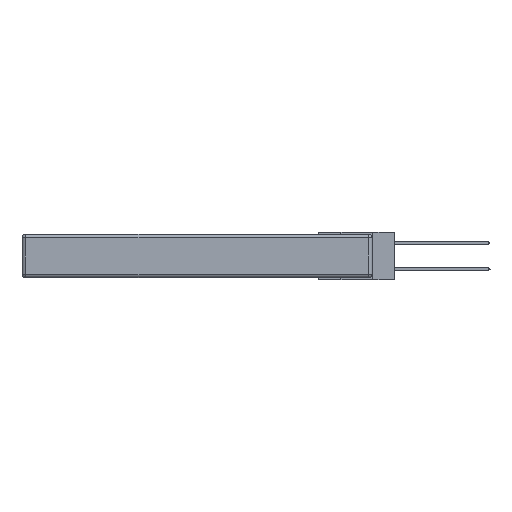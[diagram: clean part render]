
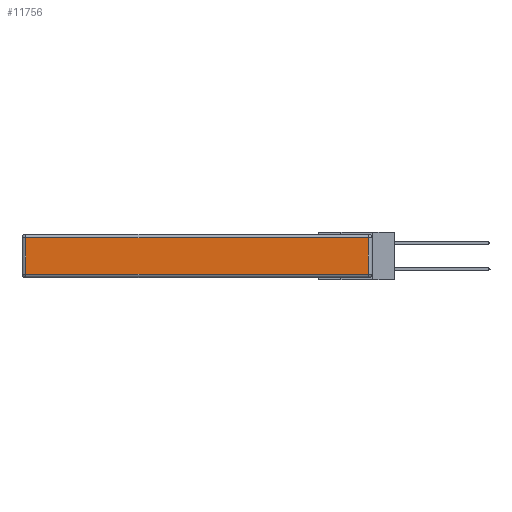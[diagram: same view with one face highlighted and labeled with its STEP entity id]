
A CAD part, left-side view. The second image highlights one B-rep face of the part: STEP entity #11756.
In plain terms, the highlighted planar face has unit normal (-1, 0, 0).
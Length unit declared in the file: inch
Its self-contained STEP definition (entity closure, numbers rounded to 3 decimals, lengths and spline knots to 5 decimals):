
#419 = ORIENTED_EDGE ( 'NONE', *, *, #9280, .T. ) ;
#491 = CARTESIAN_POINT ( 'NONE',  ( 0., 0.03, -0.03 ) ) ;
#1011 = AXIS2_PLACEMENT_3D ( 'NONE', #10241, #7585, #6358 ) ;
#1144 = CARTESIAN_POINT ( 'NONE',  ( 0., 0.03, -0.313 ) ) ;
#1223 = PLANE ( 'NONE',  #1011 ) ;
#1478 = CARTESIAN_POINT ( 'NONE',  ( 0., 2.75, -0.03 ) ) ;
#1579 = VERTEX_POINT ( 'NONE', #13434 ) ;
#1837 = DIRECTION ( 'NONE',  ( 0., 0., 1. ) ) ;
#1911 = EDGE_CURVE ( 'NONE', #4349, #9190, #3069, .T. ) ;
#3069 = LINE ( 'NONE', #1478, #7878 ) ;
#3423 = EDGE_CURVE ( 'NONE', #9190, #1579, #6467, .T. ) ;
#4105 = FACE_OUTER_BOUND ( 'NONE', #13438, .T. ) ;
#4349 = VERTEX_POINT ( 'NONE', #491 ) ;
#6188 = LINE ( 'NONE', #15758, #15163 ) ;
#6358 = DIRECTION ( 'NONE',  ( 0., 0., 1. ) ) ;
#6467 = LINE ( 'NONE', #10863, #16243 ) ;
#6690 = VECTOR ( 'NONE', #1837, 39.37008 ) ;
#7585 = DIRECTION ( 'NONE',  ( -1., 0., 0. ) ) ;
#7878 = VECTOR ( 'NONE', #10438, 39.37008 ) ;
#9190 = VERTEX_POINT ( 'NONE', #9901 ) ;
#9280 = EDGE_CURVE ( 'NONE', #1579, #16034, #6188, .T. ) ;
#9855 = ORIENTED_EDGE ( 'NONE', *, *, #3423, .T. ) ;
#9888 = LINE ( 'NONE', #12128, #6690 ) ;
#9901 = CARTESIAN_POINT ( 'NONE',  ( 0., 2.72, -0.03 ) ) ;
#10241 = CARTESIAN_POINT ( 'NONE',  ( 0., 0., -0.343 ) ) ;
#10438 = DIRECTION ( 'NONE',  ( 0., 1., 0. ) ) ;
#10863 = CARTESIAN_POINT ( 'NONE',  ( 0., 2.72, -0.343 ) ) ;
#11756 = ADVANCED_FACE ( 'NONE', ( #4105 ), #1223, .T. ) ;
#11974 = EDGE_CURVE ( 'NONE', #16034, #4349, #9888, .T. ) ;
#12128 = CARTESIAN_POINT ( 'NONE',  ( 0., 0.03, -0.343 ) ) ;
#13434 = CARTESIAN_POINT ( 'NONE',  ( 0., 2.72, -0.313 ) ) ;
#13438 = EDGE_LOOP ( 'NONE', ( #419, #15739, #14738, #9855 ) ) ;
#14571 = DIRECTION ( 'NONE',  ( 0., -1., 0. ) ) ;
#14738 = ORIENTED_EDGE ( 'NONE', *, *, #1911, .T. ) ;
#15163 = VECTOR ( 'NONE', #14571, 39.37008 ) ;
#15739 = ORIENTED_EDGE ( 'NONE', *, *, #11974, .T. ) ;
#15758 = CARTESIAN_POINT ( 'NONE',  ( 0., 0., -0.313 ) ) ;
#16034 = VERTEX_POINT ( 'NONE', #1144 ) ;
#16243 = VECTOR ( 'NONE', #16410, 39.37008 ) ;
#16410 = DIRECTION ( 'NONE',  ( 0., 0., -1. ) ) ;
